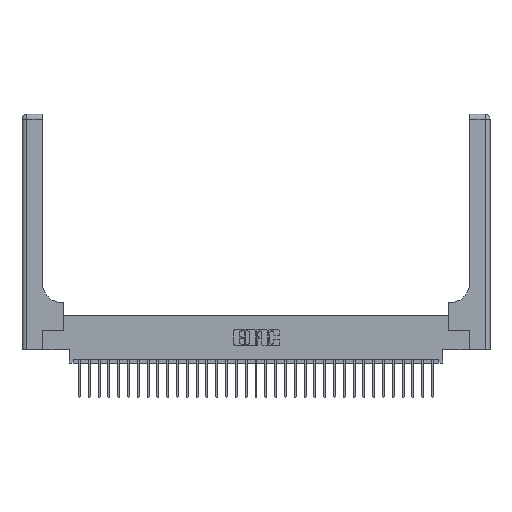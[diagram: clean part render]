
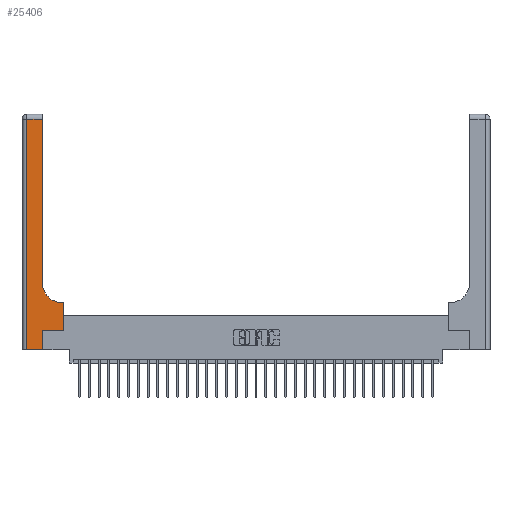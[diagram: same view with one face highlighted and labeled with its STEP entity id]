
A CAD part, top view. The second image highlights one B-rep face of the part: STEP entity #25406.
In plain terms, the highlighted planar face has unit normal (0, 0, 1).
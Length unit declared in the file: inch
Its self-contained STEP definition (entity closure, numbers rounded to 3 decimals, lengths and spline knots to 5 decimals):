
#163 = ORIENTED_EDGE ( 'NONE', *, *, #19274, .T. ) ;
#249 = CARTESIAN_POINT ( 'NONE',  ( 0.26, 0.85, 0.37 ) ) ;
#887 = VECTOR ( 'NONE', #11978, 39.37008 ) ;
#905 = CARTESIAN_POINT ( 'NONE',  ( 0.51, 0.85, 0.37 ) ) ;
#910 = EDGE_CURVE ( 'NONE', #18768, #10947, #22711, .T. ) ;
#1435 = AXIS2_PLACEMENT_3D ( 'NONE', #2072, #9072, #25392 ) ;
#1446 = EDGE_CURVE ( 'NONE', #6702, #21841, #15026, .T. ) ;
#1880 = VECTOR ( 'NONE', #23662, 39.37008 ) ;
#2072 = CARTESIAN_POINT ( 'NONE',  ( 0., 3., 0.37 ) ) ;
#2323 = CARTESIAN_POINT ( 'NONE',  ( 0.528, 0.6, 0.37 ) ) ;
#2356 = VECTOR ( 'NONE', #11125, 39.37008 ) ;
#2743 = CARTESIAN_POINT ( 'NONE',  ( 0.26, 0.6, 0.37 ) ) ;
#3053 = LINE ( 'NONE', #25746, #21625 ) ;
#3259 = DIRECTION ( 'NONE',  ( 1., 0., 0. ) ) ;
#3316 = CARTESIAN_POINT ( 'NONE',  ( 0.265, 0., 0.37 ) ) ;
#5151 = CARTESIAN_POINT ( 'NONE',  ( 0., 2.94, 0.37 ) ) ;
#6462 = ORIENTED_EDGE ( 'NONE', *, *, #13500, .T. ) ;
#6602 = LINE ( 'NONE', #7340, #1880 ) ;
#6702 = VERTEX_POINT ( 'NONE', #23264 ) ;
#6730 = PLANE ( 'NONE',  #1435 ) ;
#7340 = CARTESIAN_POINT ( 'NONE',  ( 0.265, 0.25, 0.37 ) ) ;
#7547 = EDGE_LOOP ( 'NONE', ( #29637, #21752, #163, #19253, #11685, #6462, #12139, #19159, #29910 ) ) ;
#7942 = FACE_OUTER_BOUND ( 'NONE', #7547, .T. ) ;
#8112 = CARTESIAN_POINT ( 'NONE',  ( 0.06, 3., 0.37 ) ) ;
#8146 = VECTOR ( 'NONE', #10435, 39.37008 ) ;
#8483 = VERTEX_POINT ( 'NONE', #28679 ) ;
#8514 = LINE ( 'NONE', #20425, #2356 ) ;
#9072 = DIRECTION ( 'NONE',  ( 0., 0., -1. ) ) ;
#9808 = DIRECTION ( 'NONE',  ( -1., 0., 0. ) ) ;
#10174 = CARTESIAN_POINT ( 'NONE',  ( 0.51, 0.6, 0.37 ) ) ;
#10435 = DIRECTION ( 'NONE',  ( 0., -1., 0. ) ) ;
#10947 = VERTEX_POINT ( 'NONE', #21397 ) ;
#11125 = DIRECTION ( 'NONE',  ( 0., 1., 0. ) ) ;
#11685 = ORIENTED_EDGE ( 'NONE', *, *, #11976, .T. ) ;
#11976 = EDGE_CURVE ( 'NONE', #21841, #14383, #8514, .T. ) ;
#11978 = DIRECTION ( 'NONE',  ( -1., 0., 0. ) ) ;
#12139 = ORIENTED_EDGE ( 'NONE', *, *, #21608, .T. ) ;
#13248 = LINE ( 'NONE', #2743, #887 ) ;
#13500 = EDGE_CURVE ( 'NONE', #14383, #8483, #6602, .T. ) ;
#14279 = DIRECTION ( 'NONE',  ( 1., 0., 0. ) ) ;
#14383 = VERTEX_POINT ( 'NONE', #17902 ) ;
#15026 = LINE ( 'NONE', #21322, #26744 ) ;
#16181 = CARTESIAN_POINT ( 'NONE',  ( 0.26, 2.94, 0.37 ) ) ;
#16539 = VECTOR ( 'NONE', #9808, 39.37008 ) ;
#17211 = DIRECTION ( 'NONE',  ( 0., 0., -1. ) ) ;
#17902 = CARTESIAN_POINT ( 'NONE',  ( 0.265, 0.25, 0.37 ) ) ;
#18511 = VECTOR ( 'NONE', #27498, 39.37008 ) ;
#18768 = VERTEX_POINT ( 'NONE', #16181 ) ;
#19065 = EDGE_CURVE ( 'NONE', #28414, #25772, #13248, .T. ) ;
#19159 = ORIENTED_EDGE ( 'NONE', *, *, #19065, .T. ) ;
#19253 = ORIENTED_EDGE ( 'NONE', *, *, #1446, .T. ) ;
#19274 = EDGE_CURVE ( 'NONE', #10947, #6702, #25290, .T. ) ;
#19450 = AXIS2_PLACEMENT_3D ( 'NONE', #905, #17211, #3259 ) ;
#20425 = CARTESIAN_POINT ( 'NONE',  ( 0.265, 0., 0.37 ) ) ;
#20983 = CIRCLE ( 'NONE', #19450, 0.25 ) ;
#21322 = CARTESIAN_POINT ( 'NONE',  ( 0., 0., 0.37 ) ) ;
#21397 = CARTESIAN_POINT ( 'NONE',  ( 0.06, 2.94, 0.37 ) ) ;
#21608 = EDGE_CURVE ( 'NONE', #8483, #28414, #3053, .T. ) ;
#21625 = VECTOR ( 'NONE', #28207, 39.37008 ) ;
#21752 = ORIENTED_EDGE ( 'NONE', *, *, #910, .T. ) ;
#21841 = VERTEX_POINT ( 'NONE', #3316 ) ;
#22711 = LINE ( 'NONE', #5151, #16539 ) ;
#23264 = CARTESIAN_POINT ( 'NONE',  ( 0.06, 0., 0.37 ) ) ;
#23662 = DIRECTION ( 'NONE',  ( 1., 0., 0. ) ) ;
#24721 = LINE ( 'NONE', #29738, #18511 ) ;
#25290 = LINE ( 'NONE', #8112, #8146 ) ;
#25392 = DIRECTION ( 'NONE',  ( -1., 0., 0. ) ) ;
#25406 = ADVANCED_FACE ( 'NONE', ( #7942 ), #6730, .F. ) ;
#25746 = CARTESIAN_POINT ( 'NONE',  ( 0.528, 0.25, 0.37 ) ) ;
#25772 = VERTEX_POINT ( 'NONE', #10174 ) ;
#26744 = VECTOR ( 'NONE', #14279, 39.37008 ) ;
#27498 = DIRECTION ( 'NONE',  ( 0., 1., 0. ) ) ;
#28207 = DIRECTION ( 'NONE',  ( 0., 1., 0. ) ) ;
#28265 = EDGE_CURVE ( 'NONE', #29088, #18768, #24721, .T. ) ;
#28414 = VERTEX_POINT ( 'NONE', #2323 ) ;
#28679 = CARTESIAN_POINT ( 'NONE',  ( 0.528, 0.25, 0.37 ) ) ;
#29088 = VERTEX_POINT ( 'NONE', #249 ) ;
#29637 = ORIENTED_EDGE ( 'NONE', *, *, #28265, .T. ) ;
#29738 = CARTESIAN_POINT ( 'NONE',  ( 0.26, 3., 0.37 ) ) ;
#29874 = EDGE_CURVE ( 'NONE', #25772, #29088, #20983, .T. ) ;
#29910 = ORIENTED_EDGE ( 'NONE', *, *, #29874, .T. ) ;
